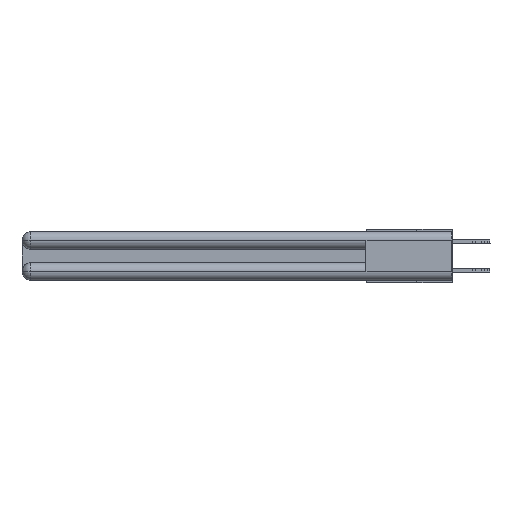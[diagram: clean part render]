
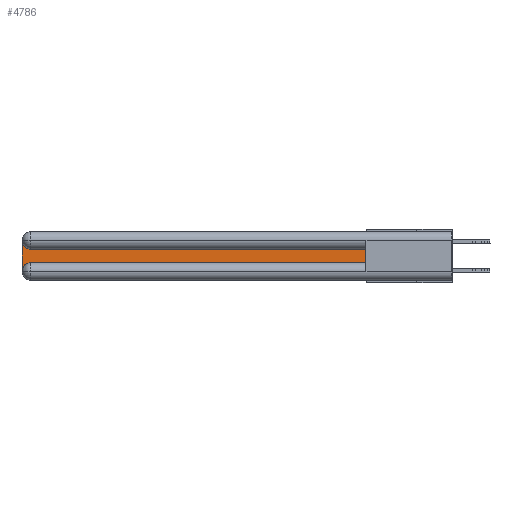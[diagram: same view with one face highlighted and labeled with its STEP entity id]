
A CAD part, left-side view. The second image highlights one B-rep face of the part: STEP entity #4786.
In plain terms, the highlighted planar face has unit normal (-1, 0, 0).
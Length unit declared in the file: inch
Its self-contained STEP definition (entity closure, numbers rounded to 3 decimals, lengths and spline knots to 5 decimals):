
#204 = EDGE_CURVE ( 'NONE', #16050, #17916, #3668, .T. ) ;
#1807 = DIRECTION ( 'NONE',  ( 0., 0., -1. ) ) ;
#1948 = CARTESIAN_POINT ( 'NONE',  ( 0.075, 0.6, -0.2175 ) ) ;
#3668 = CIRCLE ( 'NONE', #13340, 0.06 ) ;
#3726 = VERTEX_POINT ( 'NONE', #30258 ) ;
#3833 = CARTESIAN_POINT ( 'NONE',  ( 0.075, 2.94, -0.2175 ) ) ;
#4044 = DIRECTION ( 'NONE',  ( 1., 0., 0. ) ) ;
#4344 = CARTESIAN_POINT ( 'NONE',  ( 0.075, 0.6, -0.1225 ) ) ;
#4351 = ORIENTED_EDGE ( 'NONE', *, *, #204, .T. ) ;
#4786 = ADVANCED_FACE ( 'NONE', ( #30274 ), #24478, .F. ) ;
#5244 = EDGE_CURVE ( 'NONE', #27873, #31086, #30244, .T. ) ;
#5758 = ORIENTED_EDGE ( 'NONE', *, *, #22591, .T. ) ;
#6365 = ORIENTED_EDGE ( 'NONE', *, *, #8975, .T. ) ;
#6628 = CARTESIAN_POINT ( 'NONE',  ( 0.075, 3., -0.1225 ) ) ;
#7566 = EDGE_CURVE ( 'NONE', #31086, #9604, #27671, .T. ) ;
#7717 = DIRECTION ( 'NONE',  ( 0., 1., 0. ) ) ;
#8975 = EDGE_CURVE ( 'NONE', #17916, #27873, #30374, .T. ) ;
#9081 = VECTOR ( 'NONE', #1807, 39.37008 ) ;
#9604 = VERTEX_POINT ( 'NONE', #31719 ) ;
#10904 = AXIS2_PLACEMENT_3D ( 'NONE', #29505, #13835, #21692 ) ;
#13189 = CARTESIAN_POINT ( 'NONE',  ( 0.075, 2.94, -0.2775 ) ) ;
#13340 = AXIS2_PLACEMENT_3D ( 'NONE', #13189, #31607, #31489 ) ;
#13835 = DIRECTION ( 'NONE',  ( 1., 0., 0. ) ) ;
#15057 = CARTESIAN_POINT ( 'NONE',  ( 0.075, 0.6, -0.2175 ) ) ;
#16050 = VERTEX_POINT ( 'NONE', #23999 ) ;
#16455 = LINE ( 'NONE', #17777, #9081 ) ;
#17703 = DIRECTION ( 'NONE',  ( 0., -1., 0. ) ) ;
#17736 = CARTESIAN_POINT ( 'NONE',  ( 0.075, 0.6, -0.2175 ) ) ;
#17777 = CARTESIAN_POINT ( 'NONE',  ( 0.075, 3., -0.2175 ) ) ;
#17916 = VERTEX_POINT ( 'NONE', #3833 ) ;
#17917 = DIRECTION ( 'NONE',  ( 0., 0., 1. ) ) ;
#19797 = AXIS2_PLACEMENT_3D ( 'NONE', #6628, #4044, #22177 ) ;
#20004 = CIRCLE ( 'NONE', #10904, 0.06 ) ;
#20035 = EDGE_LOOP ( 'NONE', ( #27184, #24481, #5758, #4351, #6365, #31968 ) ) ;
#20690 = VECTOR ( 'NONE', #7717, 39.37008 ) ;
#21221 = VECTOR ( 'NONE', #17917, 39.37008 ) ;
#21692 = DIRECTION ( 'NONE',  ( 0., 0., -1. ) ) ;
#22177 = DIRECTION ( 'NONE',  ( 0., 0., -1. ) ) ;
#22591 = EDGE_CURVE ( 'NONE', #3726, #16050, #16455, .T. ) ;
#23363 = CARTESIAN_POINT ( 'NONE',  ( 0.075, 0.6, -0.1225 ) ) ;
#23999 = CARTESIAN_POINT ( 'NONE',  ( 0.075, 3., -0.2775 ) ) ;
#24478 = PLANE ( 'NONE',  #19797 ) ;
#24481 = ORIENTED_EDGE ( 'NONE', *, *, #30921, .T. ) ;
#26247 = VECTOR ( 'NONE', #17703, 39.37008 ) ;
#27184 = ORIENTED_EDGE ( 'NONE', *, *, #7566, .T. ) ;
#27671 = LINE ( 'NONE', #23363, #20690 ) ;
#27873 = VERTEX_POINT ( 'NONE', #17736 ) ;
#29505 = CARTESIAN_POINT ( 'NONE',  ( 0.075, 2.94, -0.0625 ) ) ;
#30244 = LINE ( 'NONE', #1948, #21221 ) ;
#30258 = CARTESIAN_POINT ( 'NONE',  ( 0.075, 3., -0.0625 ) ) ;
#30274 = FACE_OUTER_BOUND ( 'NONE', #20035, .T. ) ;
#30374 = LINE ( 'NONE', #15057, #26247 ) ;
#30921 = EDGE_CURVE ( 'NONE', #9604, #3726, #20004, .T. ) ;
#31086 = VERTEX_POINT ( 'NONE', #4344 ) ;
#31489 = DIRECTION ( 'NONE',  ( 0., 0., -1. ) ) ;
#31607 = DIRECTION ( 'NONE',  ( 1., 0., 0. ) ) ;
#31719 = CARTESIAN_POINT ( 'NONE',  ( 0.075, 2.94, -0.1225 ) ) ;
#31968 = ORIENTED_EDGE ( 'NONE', *, *, #5244, .T. ) ;
